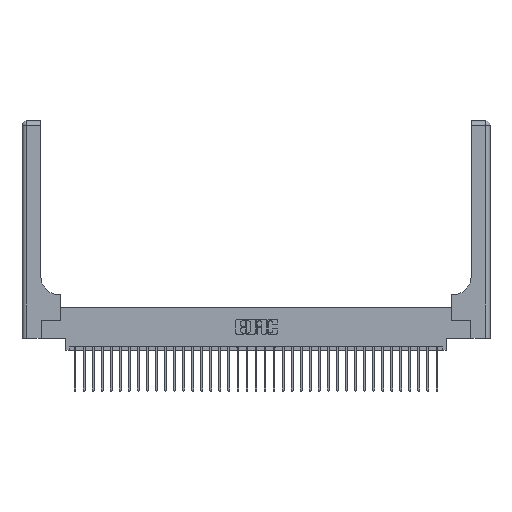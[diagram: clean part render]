
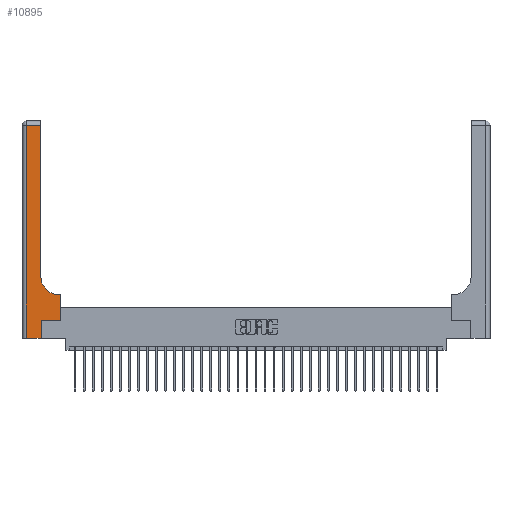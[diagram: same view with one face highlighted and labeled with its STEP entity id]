
A CAD part, top view. The second image highlights one B-rep face of the part: STEP entity #10895.
In plain terms, the highlighted planar face has unit normal (0, 0, 1).
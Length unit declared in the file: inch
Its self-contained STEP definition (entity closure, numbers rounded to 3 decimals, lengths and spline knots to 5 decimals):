
#235 = CARTESIAN_POINT ( 'NONE',  ( 0.528, 0.25, 0.37 ) ) ;
#1274 = CARTESIAN_POINT ( 'NONE',  ( 0.528, 0.6, 0.37 ) ) ;
#1818 = VECTOR ( 'NONE', #31667, 39.37008 ) ;
#2353 = ORIENTED_EDGE ( 'NONE', *, *, #24938, .T. ) ;
#2766 = CARTESIAN_POINT ( 'NONE',  ( 0.26, 3., 0.37 ) ) ;
#2784 = ORIENTED_EDGE ( 'NONE', *, *, #17709, .T. ) ;
#2785 = VECTOR ( 'NONE', #26955, 39.37008 ) ;
#2951 = CARTESIAN_POINT ( 'NONE',  ( 0.528, 0.25, 0.37 ) ) ;
#3462 = EDGE_CURVE ( 'NONE', #12403, #26439, #9391, .T. ) ;
#3527 = AXIS2_PLACEMENT_3D ( 'NONE', #26463, #19071, #4166 ) ;
#4119 = LINE ( 'NONE', #19981, #16570 ) ;
#4151 = EDGE_CURVE ( 'NONE', #28018, #28992, #22235, .T. ) ;
#4166 = DIRECTION ( 'NONE',  ( -1., 0., 0. ) ) ;
#5168 = CARTESIAN_POINT ( 'NONE',  ( 0.265, 0., 0.37 ) ) ;
#5252 = ORIENTED_EDGE ( 'NONE', *, *, #7947, .T. ) ;
#5851 = CARTESIAN_POINT ( 'NONE',  ( 0.06, 2.94, 0.37 ) ) ;
#6628 = VERTEX_POINT ( 'NONE', #15395 ) ;
#7006 = EDGE_CURVE ( 'NONE', #13095, #15400, #21702, .T. ) ;
#7369 = CARTESIAN_POINT ( 'NONE',  ( 0.06, 0., 0.37 ) ) ;
#7839 = DIRECTION ( 'NONE',  ( 0., 0., -1. ) ) ;
#7843 = DIRECTION ( 'NONE',  ( 0., 1., 0. ) ) ;
#7947 = EDGE_CURVE ( 'NONE', #15400, #12403, #4119, .T. ) ;
#8951 = VECTOR ( 'NONE', #30071, 39.37008 ) ;
#9391 = LINE ( 'NONE', #12049, #2785 ) ;
#10038 = DIRECTION ( 'NONE',  ( 1., 0., 0. ) ) ;
#10895 = ADVANCED_FACE ( 'NONE', ( #13253 ), #11530, .F. ) ;
#11530 = PLANE ( 'NONE',  #3527 ) ;
#12049 = CARTESIAN_POINT ( 'NONE',  ( 0.265, 0., 0.37 ) ) ;
#12403 = VERTEX_POINT ( 'NONE', #5168 ) ;
#12736 = CARTESIAN_POINT ( 'NONE',  ( 0.51, 0.6, 0.37 ) ) ;
#13095 = VERTEX_POINT ( 'NONE', #5851 ) ;
#13253 = FACE_OUTER_BOUND ( 'NONE', #27168, .T. ) ;
#14260 = EDGE_CURVE ( 'NONE', #23112, #28018, #25097, .T. ) ;
#14792 = CARTESIAN_POINT ( 'NONE',  ( 0.265, 0.25, 0.37 ) ) ;
#15104 = VERTEX_POINT ( 'NONE', #21321 ) ;
#15395 = CARTESIAN_POINT ( 'NONE',  ( 0.26, 0.85, 0.37 ) ) ;
#15400 = VERTEX_POINT ( 'NONE', #7369 ) ;
#16570 = VECTOR ( 'NONE', #10038, 39.37008 ) ;
#16713 = CARTESIAN_POINT ( 'NONE',  ( 0., 2.94, 0.37 ) ) ;
#16744 = ORIENTED_EDGE ( 'NONE', *, *, #3462, .T. ) ;
#17646 = ORIENTED_EDGE ( 'NONE', *, *, #24637, .T. ) ;
#17709 = EDGE_CURVE ( 'NONE', #15104, #13095, #24392, .T. ) ;
#17882 = ORIENTED_EDGE ( 'NONE', *, *, #14260, .T. ) ;
#18584 = EDGE_CURVE ( 'NONE', #28992, #6628, #20840, .T. ) ;
#19071 = DIRECTION ( 'NONE',  ( 0., 0., -1. ) ) ;
#19087 = AXIS2_PLACEMENT_3D ( 'NONE', #22770, #7839, #25267 ) ;
#19155 = ORIENTED_EDGE ( 'NONE', *, *, #4151, .T. ) ;
#19981 = CARTESIAN_POINT ( 'NONE',  ( 0., 0., 0.37 ) ) ;
#20248 = ORIENTED_EDGE ( 'NONE', *, *, #18584, .T. ) ;
#20840 = CIRCLE ( 'NONE', #19087, 0.25 ) ;
#21321 = CARTESIAN_POINT ( 'NONE',  ( 0.26, 2.94, 0.37 ) ) ;
#21621 = DIRECTION ( 'NONE',  ( 1., 0., 0. ) ) ;
#21702 = LINE ( 'NONE', #29135, #1818 ) ;
#22235 = LINE ( 'NONE', #24528, #22995 ) ;
#22770 = CARTESIAN_POINT ( 'NONE',  ( 0.51, 0.85, 0.37 ) ) ;
#22995 = VECTOR ( 'NONE', #29512, 39.37008 ) ;
#23112 = VERTEX_POINT ( 'NONE', #235 ) ;
#23413 = VECTOR ( 'NONE', #21621, 39.37008 ) ;
#24309 = VECTOR ( 'NONE', #7843, 39.37008 ) ;
#24392 = LINE ( 'NONE', #16713, #30976 ) ;
#24528 = CARTESIAN_POINT ( 'NONE',  ( 0.26, 0.6, 0.37 ) ) ;
#24637 = EDGE_CURVE ( 'NONE', #26439, #23112, #30023, .T. ) ;
#24938 = EDGE_CURVE ( 'NONE', #6628, #15104, #28803, .T. ) ;
#25097 = LINE ( 'NONE', #2951, #24309 ) ;
#25267 = DIRECTION ( 'NONE',  ( 1., 0., 0. ) ) ;
#26439 = VERTEX_POINT ( 'NONE', #14792 ) ;
#26463 = CARTESIAN_POINT ( 'NONE',  ( 0., 3., 0.37 ) ) ;
#26955 = DIRECTION ( 'NONE',  ( 0., 1., 0. ) ) ;
#27168 = EDGE_LOOP ( 'NONE', ( #2353, #2784, #30642, #5252, #16744, #17646, #17882, #19155, #20248 ) ) ;
#28018 = VERTEX_POINT ( 'NONE', #1274 ) ;
#28803 = LINE ( 'NONE', #2766, #8951 ) ;
#28967 = CARTESIAN_POINT ( 'NONE',  ( 0.265, 0.25, 0.37 ) ) ;
#28992 = VERTEX_POINT ( 'NONE', #12736 ) ;
#29135 = CARTESIAN_POINT ( 'NONE',  ( 0.06, 3., 0.37 ) ) ;
#29512 = DIRECTION ( 'NONE',  ( -1., 0., 0. ) ) ;
#30023 = LINE ( 'NONE', #28967, #23413 ) ;
#30071 = DIRECTION ( 'NONE',  ( 0., 1., 0. ) ) ;
#30642 = ORIENTED_EDGE ( 'NONE', *, *, #7006, .T. ) ;
#30976 = VECTOR ( 'NONE', #31601, 39.37008 ) ;
#31601 = DIRECTION ( 'NONE',  ( -1., 0., 0. ) ) ;
#31667 = DIRECTION ( 'NONE',  ( 0., -1., 0. ) ) ;
